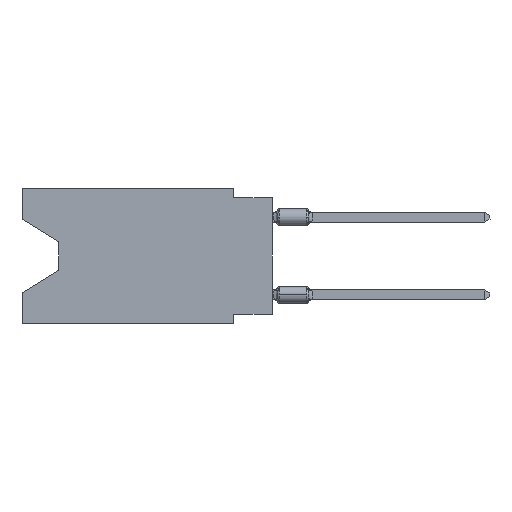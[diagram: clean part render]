
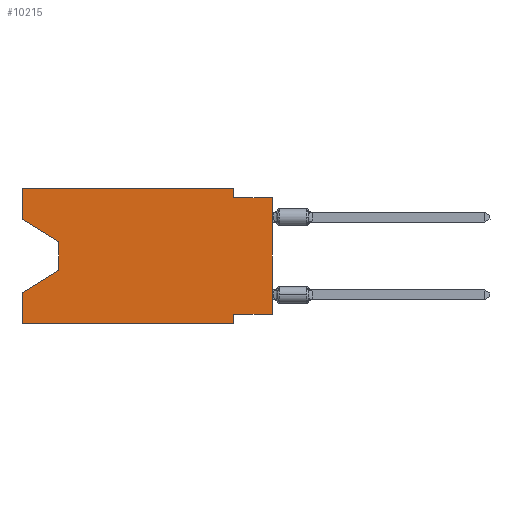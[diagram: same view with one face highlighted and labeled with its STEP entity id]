
A CAD part, left-side view. The second image highlights one B-rep face of the part: STEP entity #10215.
In plain terms, the highlighted planar face has unit normal (-1, 0, 0).
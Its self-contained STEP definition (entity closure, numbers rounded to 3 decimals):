
#309 = EDGE_CURVE ( 'NONE', #18035, #418, #10145, .T. ) ;
#394 = CARTESIAN_POINT ( 'NONE',  ( 0., 0., -0.635 ) ) ;
#418 = VERTEX_POINT ( 'NONE', #13398 ) ;
#511 = CARTESIAN_POINT ( 'NONE',  ( 0., 16.383, 0. ) ) ;
#956 = CARTESIAN_POINT ( 'NONE',  ( 0., 2.54, -8.255 ) ) ;
#1275 = VERTEX_POINT ( 'NONE', #14205 ) ;
#1421 = VECTOR ( 'NONE', #4575, 1000. ) ;
#1764 = VERTEX_POINT ( 'NONE', #8048 ) ;
#1784 = VECTOR ( 'NONE', #14841, 1000. ) ;
#1982 = VERTEX_POINT ( 'NONE', #8560 ) ;
#2105 = ORIENTED_EDGE ( 'NONE', *, *, #15035, .F. ) ;
#2112 = PLANE ( 'NONE',  #12970 ) ;
#2264 = ORIENTED_EDGE ( 'NONE', *, *, #9309, .T. ) ;
#2823 = CARTESIAN_POINT ( 'NONE',  ( 0., 16.383, 0. ) ) ;
#3023 = LINE ( 'NONE', #10397, #17970 ) ;
#3131 = DIRECTION ( 'NONE',  ( 0., 0., 1. ) ) ;
#3343 = VECTOR ( 'NONE', #11740, 1000. ) ;
#3987 = VERTEX_POINT ( 'NONE', #5516 ) ;
#3997 = CARTESIAN_POINT ( 'NONE',  ( 0., 16.383, 0. ) ) ;
#4115 = LINE ( 'NONE', #2823, #12259 ) ;
#4575 = DIRECTION ( 'NONE',  ( 0., -1., 0. ) ) ;
#4588 = VERTEX_POINT ( 'NONE', #6654 ) ;
#4846 = LINE ( 'NONE', #10914, #12628 ) ;
#4884 = DIRECTION ( 'NONE',  ( 0., 0., 1. ) ) ;
#4992 = VECTOR ( 'NONE', #7815, 1000. ) ;
#5035 = LINE ( 'NONE', #6331, #5314 ) ;
#5086 = ORIENTED_EDGE ( 'NONE', *, *, #10051, .F. ) ;
#5314 = VECTOR ( 'NONE', #9423, 1000. ) ;
#5433 = EDGE_CURVE ( 'NONE', #11508, #1764, #16836, .T. ) ;
#5516 = CARTESIAN_POINT ( 'NONE',  ( 0., 16.383, -6.852 ) ) ;
#6292 = CARTESIAN_POINT ( 'NONE',  ( 0., 16.383, 0. ) ) ;
#6331 = CARTESIAN_POINT ( 'NONE',  ( 0., 2.54, -8.89 ) ) ;
#6386 = LINE ( 'NONE', #6292, #9784 ) ;
#6654 = CARTESIAN_POINT ( 'NONE',  ( 0., 2.54, -0.635 ) ) ;
#6684 = VERTEX_POINT ( 'NONE', #3997 ) ;
#7411 = EDGE_CURVE ( 'NONE', #13327, #4588, #16892, .T. ) ;
#7436 = LINE ( 'NONE', #19122, #3343 ) ;
#7684 = ORIENTED_EDGE ( 'NONE', *, *, #11626, .F. ) ;
#7714 = DIRECTION ( 'NONE',  ( 0., 0.855, -0.519 ) ) ;
#7815 = DIRECTION ( 'NONE',  ( 0., -1., 0. ) ) ;
#7869 = CARTESIAN_POINT ( 'NONE',  ( 0., 0., 0. ) ) ;
#8048 = CARTESIAN_POINT ( 'NONE',  ( 0., 0., -0.635 ) ) ;
#8155 = VECTOR ( 'NONE', #13900, 1000. ) ;
#8214 = DIRECTION ( 'NONE',  ( 0., -1., 0. ) ) ;
#8438 = CARTESIAN_POINT ( 'NONE',  ( 0., 16.383, -2.038 ) ) ;
#8560 = CARTESIAN_POINT ( 'NONE',  ( 0., 2.54, -8.89 ) ) ;
#9208 = ORIENTED_EDGE ( 'NONE', *, *, #9263, .T. ) ;
#9263 = EDGE_CURVE ( 'NONE', #19615, #3987, #4846, .T. ) ;
#9309 = EDGE_CURVE ( 'NONE', #1275, #1982, #12423, .T. ) ;
#9423 = DIRECTION ( 'NONE',  ( 0., 0., -1. ) ) ;
#9464 = VECTOR ( 'NONE', #13024, 1000. ) ;
#9666 = ORIENTED_EDGE ( 'NONE', *, *, #15007, .F. ) ;
#9784 = VECTOR ( 'NONE', #3131, 1000. ) ;
#10051 = EDGE_CURVE ( 'NONE', #18035, #6684, #6386, .T. ) ;
#10145 = LINE ( 'NONE', #13206, #9464 ) ;
#10215 = ADVANCED_FACE ( 'NONE', ( #17231 ), #2112, .F. ) ;
#10300 = ORIENTED_EDGE ( 'NONE', *, *, #309, .T. ) ;
#10397 = CARTESIAN_POINT ( 'NONE',  ( 0., 16.383, 0. ) ) ;
#10437 = EDGE_LOOP ( 'NONE', ( #10300, #12033, #9208, #13883, #2264, #10515, #2105, #11432, #7684, #12330, #9666, #5086 ) ) ;
#10515 = ORIENTED_EDGE ( 'NONE', *, *, #16122, .F. ) ;
#10914 = CARTESIAN_POINT ( 'NONE',  ( 0., 13.97, -5.385 ) ) ;
#11116 = CARTESIAN_POINT ( 'NONE',  ( 0., 13.97, -5.385 ) ) ;
#11432 = ORIENTED_EDGE ( 'NONE', *, *, #5433, .T. ) ;
#11508 = VERTEX_POINT ( 'NONE', #13149 ) ;
#11626 = EDGE_CURVE ( 'NONE', #4588, #1764, #15523, .T. ) ;
#11740 = DIRECTION ( 'NONE',  ( 0., 0., -1. ) ) ;
#11881 = EDGE_CURVE ( 'NONE', #418, #19615, #7436, .T. ) ;
#12033 = ORIENTED_EDGE ( 'NONE', *, *, #11881, .T. ) ;
#12259 = VECTOR ( 'NONE', #8214, 1000. ) ;
#12330 = ORIENTED_EDGE ( 'NONE', *, *, #7411, .F. ) ;
#12388 = EDGE_CURVE ( 'NONE', #1275, #3987, #3023, .T. ) ;
#12423 = LINE ( 'NONE', #15282, #4992 ) ;
#12628 = VECTOR ( 'NONE', #7714, 1000. ) ;
#12665 = DIRECTION ( 'NONE',  ( 1., 0., 0. ) ) ;
#12970 = AXIS2_PLACEMENT_3D ( 'NONE', #511, #12665, #18755 ) ;
#13024 = DIRECTION ( 'NONE',  ( 0., -0.855, -0.519 ) ) ;
#13149 = CARTESIAN_POINT ( 'NONE',  ( 0., 0., -8.255 ) ) ;
#13206 = CARTESIAN_POINT ( 'NONE',  ( 0., 16.383, -2.038 ) ) ;
#13327 = VERTEX_POINT ( 'NONE', #17566 ) ;
#13398 = CARTESIAN_POINT ( 'NONE',  ( 0., 13.97, -3.505 ) ) ;
#13883 = ORIENTED_EDGE ( 'NONE', *, *, #12388, .F. ) ;
#13900 = DIRECTION ( 'NONE',  ( 0., 0., -1. ) ) ;
#14205 = CARTESIAN_POINT ( 'NONE',  ( 0., 16.383, -8.89 ) ) ;
#14736 = LINE ( 'NONE', #16333, #1784 ) ;
#14841 = DIRECTION ( 'NONE',  ( 0., 1., 0. ) ) ;
#15007 = EDGE_CURVE ( 'NONE', #6684, #13327, #4115, .T. ) ;
#15035 = EDGE_CURVE ( 'NONE', #11508, #18463, #14736, .T. ) ;
#15282 = CARTESIAN_POINT ( 'NONE',  ( 0., 16.383, -8.89 ) ) ;
#15283 = CARTESIAN_POINT ( 'NONE',  ( 0., 2.54, 0. ) ) ;
#15523 = LINE ( 'NONE', #394, #1421 ) ;
#16122 = EDGE_CURVE ( 'NONE', #18463, #1982, #5035, .T. ) ;
#16333 = CARTESIAN_POINT ( 'NONE',  ( 0., 0., -8.255 ) ) ;
#16554 = DIRECTION ( 'NONE',  ( 0., 0., 1. ) ) ;
#16836 = LINE ( 'NONE', #7869, #18105 ) ;
#16892 = LINE ( 'NONE', #15283, #8155 ) ;
#17231 = FACE_OUTER_BOUND ( 'NONE', #10437, .T. ) ;
#17566 = CARTESIAN_POINT ( 'NONE',  ( 0., 2.54, 0. ) ) ;
#17970 = VECTOR ( 'NONE', #16554, 1000. ) ;
#18035 = VERTEX_POINT ( 'NONE', #8438 ) ;
#18105 = VECTOR ( 'NONE', #4884, 1000. ) ;
#18463 = VERTEX_POINT ( 'NONE', #956 ) ;
#18755 = DIRECTION ( 'NONE',  ( 0., 0., -1. ) ) ;
#19122 = CARTESIAN_POINT ( 'NONE',  ( 0., 13.97, -3.505 ) ) ;
#19615 = VERTEX_POINT ( 'NONE', #11116 ) ;
